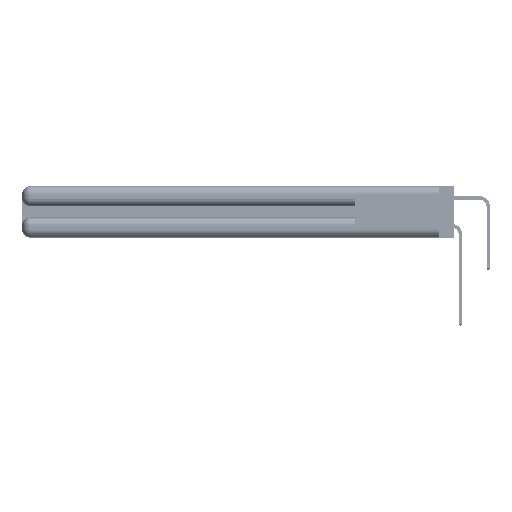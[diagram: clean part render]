
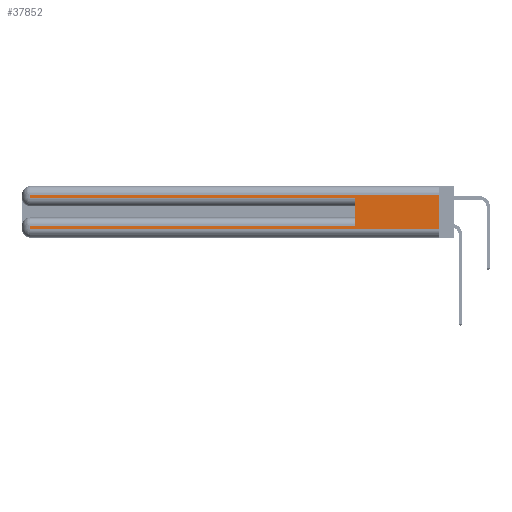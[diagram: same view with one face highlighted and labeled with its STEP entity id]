
A CAD part, left-side view. The second image highlights one B-rep face of the part: STEP entity #37852.
In plain terms, the highlighted planar face has unit normal (-1, 0, 0).
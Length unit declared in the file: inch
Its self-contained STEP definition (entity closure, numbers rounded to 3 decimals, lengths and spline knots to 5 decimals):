
#1364 = ORIENTED_EDGE ( 'NONE', *, *, #9000, .T. ) ;
#2700 = VECTOR ( 'NONE', #25176, 39.37008 ) ;
#4609 = EDGE_CURVE ( 'NONE', #30601, #16610, #39098, .T. ) ;
#5634 = ORIENTED_EDGE ( 'NONE', *, *, #42853, .T. ) ;
#6091 = CARTESIAN_POINT ( 'NONE',  ( 0., 0., 0.37 ) ) ;
#6849 = VECTOR ( 'NONE', #27099, 39.37008 ) ;
#6930 = CARTESIAN_POINT ( 'NONE',  ( 0., 0.6, 0.145 ) ) ;
#7000 = EDGE_CURVE ( 'NONE', #23579, #23852, #36288, .T. ) ;
#9000 = EDGE_CURVE ( 'NONE', #13546, #23579, #32676, .T. ) ;
#9218 = VECTOR ( 'NONE', #11682, 39.37008 ) ;
#9670 = DIRECTION ( 'NONE',  ( 0., -1., 0. ) ) ;
#10140 = DIRECTION ( 'NONE',  ( 0., 0., -1. ) ) ;
#10982 = VECTOR ( 'NONE', #18896, 39.37008 ) ;
#11682 = DIRECTION ( 'NONE',  ( 0., -1., 0. ) ) ;
#13516 = LINE ( 'NONE', #41522, #33754 ) ;
#13546 = VERTEX_POINT ( 'NONE', #38778 ) ;
#14392 = CARTESIAN_POINT ( 'NONE',  ( 0., 0., 0.06 ) ) ;
#16610 = VERTEX_POINT ( 'NONE', #47766 ) ;
#17921 = CARTESIAN_POINT ( 'NONE',  ( 0., 0., 0.37 ) ) ;
#18308 = EDGE_LOOP ( 'NONE', ( #18899, #43599, #5634, #49292, #51846, #48727, #1364, #47517 ) ) ;
#18896 = DIRECTION ( 'NONE',  ( 0., 1., 0. ) ) ;
#18899 = ORIENTED_EDGE ( 'NONE', *, *, #19465, .F. ) ;
#19465 = EDGE_CURVE ( 'NONE', #30773, #23852, #51864, .T. ) ;
#22048 = DIRECTION ( 'NONE',  ( 0., 0., -1. ) ) ;
#23449 = CARTESIAN_POINT ( 'NONE',  ( 0., 0., 0.31 ) ) ;
#23579 = VERTEX_POINT ( 'NONE', #40398 ) ;
#23852 = VERTEX_POINT ( 'NONE', #14392 ) ;
#24316 = VECTOR ( 'NONE', #9670, 39.37008 ) ;
#24592 = EDGE_CURVE ( 'NONE', #46863, #16610, #33248, .T. ) ;
#25176 = DIRECTION ( 'NONE',  ( 0., 1., 0. ) ) ;
#27099 = DIRECTION ( 'NONE',  ( 0., 0., 1. ) ) ;
#27777 = CARTESIAN_POINT ( 'NONE',  ( 0., 0., 0.285 ) ) ;
#29814 = CARTESIAN_POINT ( 'NONE',  ( 0., 0., 0.06 ) ) ;
#30272 = PLANE ( 'NONE',  #35563 ) ;
#30426 = VECTOR ( 'NONE', #22048, 39.37008 ) ;
#30581 = FACE_OUTER_BOUND ( 'NONE', #18308, .T. ) ;
#30601 = VERTEX_POINT ( 'NONE', #34403 ) ;
#30773 = VERTEX_POINT ( 'NONE', #23449 ) ;
#31210 = LINE ( 'NONE', #43123, #10982 ) ;
#31389 = VECTOR ( 'NONE', #49164, 39.37008 ) ;
#32676 = LINE ( 'NONE', #37164, #31389 ) ;
#33248 = LINE ( 'NONE', #27777, #9218 ) ;
#33677 = LINE ( 'NONE', #49351, #2700 ) ;
#33754 = VECTOR ( 'NONE', #45576, 39.37008 ) ;
#33775 = CARTESIAN_POINT ( 'NONE',  ( 0., 2.94, 0.31 ) ) ;
#34340 = DIRECTION ( 'NONE',  ( 1., 0., 0. ) ) ;
#34403 = CARTESIAN_POINT ( 'NONE',  ( 0., 0.6, 0.085 ) ) ;
#35563 = AXIS2_PLACEMENT_3D ( 'NONE', #6091, #34340, #10140 ) ;
#36288 = LINE ( 'NONE', #29814, #24316 ) ;
#37164 = CARTESIAN_POINT ( 'NONE',  ( 0., 2.94, 0.37 ) ) ;
#37735 = CARTESIAN_POINT ( 'NONE',  ( 0., 2.94, 0.285 ) ) ;
#37852 = ADVANCED_FACE ( 'NONE', ( #30581 ), #30272, .F. ) ;
#38441 = EDGE_CURVE ( 'NONE', #30773, #51432, #33677, .T. ) ;
#38778 = CARTESIAN_POINT ( 'NONE',  ( 0., 2.94, 0.085 ) ) ;
#39098 = LINE ( 'NONE', #6930, #6849 ) ;
#40398 = CARTESIAN_POINT ( 'NONE',  ( 0., 2.94, 0.06 ) ) ;
#41522 = CARTESIAN_POINT ( 'NONE',  ( 0., 2.94, 0.37 ) ) ;
#42853 = EDGE_CURVE ( 'NONE', #51432, #46863, #13516, .T. ) ;
#43123 = CARTESIAN_POINT ( 'NONE',  ( 0., 0., 0.085 ) ) ;
#43599 = ORIENTED_EDGE ( 'NONE', *, *, #38441, .T. ) ;
#45576 = DIRECTION ( 'NONE',  ( 0., 0., -1. ) ) ;
#46863 = VERTEX_POINT ( 'NONE', #37735 ) ;
#47517 = ORIENTED_EDGE ( 'NONE', *, *, #7000, .T. ) ;
#47766 = CARTESIAN_POINT ( 'NONE',  ( 0., 0.6, 0.285 ) ) ;
#47911 = EDGE_CURVE ( 'NONE', #30601, #13546, #31210, .T. ) ;
#48727 = ORIENTED_EDGE ( 'NONE', *, *, #47911, .T. ) ;
#49164 = DIRECTION ( 'NONE',  ( 0., 0., -1. ) ) ;
#49292 = ORIENTED_EDGE ( 'NONE', *, *, #24592, .T. ) ;
#49351 = CARTESIAN_POINT ( 'NONE',  ( 0., 0., 0.31 ) ) ;
#51432 = VERTEX_POINT ( 'NONE', #33775 ) ;
#51846 = ORIENTED_EDGE ( 'NONE', *, *, #4609, .F. ) ;
#51864 = LINE ( 'NONE', #17921, #30426 ) ;
